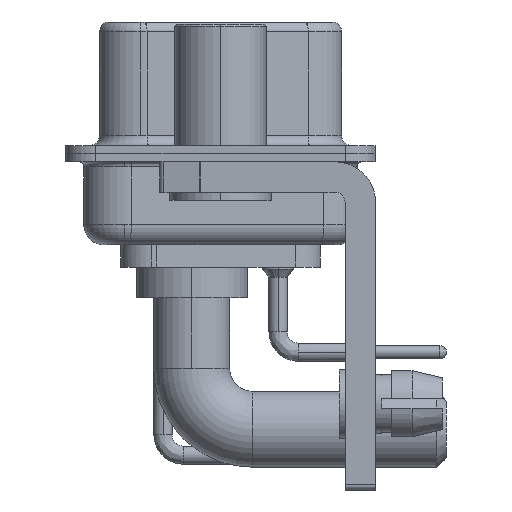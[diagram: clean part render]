
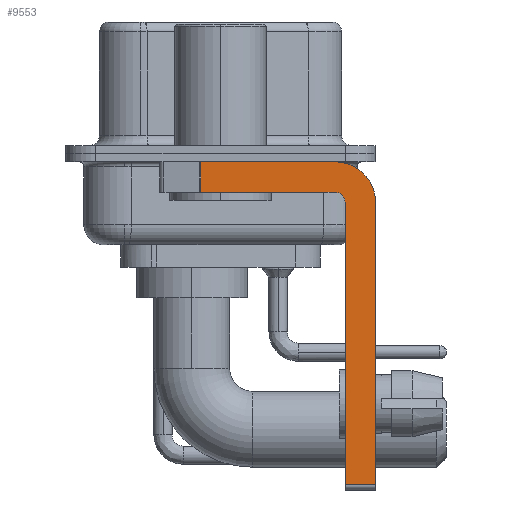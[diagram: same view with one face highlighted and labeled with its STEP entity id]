
A CAD part, left-side view. The second image highlights one B-rep face of the part: STEP entity #9553.
In plain terms, the highlighted planar face has unit normal (-1, 0, 0).
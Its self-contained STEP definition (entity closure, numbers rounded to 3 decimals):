
#256 = DIRECTION ( 'NONE',  ( 0., 0., -1. ) ) ;
#815 = LINE ( 'NONE', #10758, #29738 ) ;
#820 = VERTEX_POINT ( 'NONE', #36194 ) ;
#2617 = CARTESIAN_POINT ( 'NONE',  ( -2.9, 3., -0.4 ) ) ;
#3922 = CARTESIAN_POINT ( 'NONE',  ( -2.9, 0.978, -1.9 ) ) ;
#4291 = CIRCLE ( 'NONE', #25644, 2. ) ;
#4323 = CARTESIAN_POINT ( 'NONE',  ( -2.9, -5.65, -2.4 ) ) ;
#5195 = VERTEX_POINT ( 'NONE', #13333 ) ;
#5649 = CARTESIAN_POINT ( 'NONE',  ( -2.9, -7.65, -2.4 ) ) ;
#6351 = EDGE_CURVE ( 'NONE', #15747, #5195, #4291, .T. ) ;
#7833 = AXIS2_PLACEMENT_3D ( 'NONE', #21275, #9459, #33469 ) ;
#8758 = LINE ( 'NONE', #2617, #20446 ) ;
#9337 = VERTEX_POINT ( 'NONE', #18661 ) ;
#9459 = DIRECTION ( 'NONE',  ( 1., 0., 0. ) ) ;
#9553 = ADVANCED_FACE ( 'NONE', ( #19042 ), #27560, .F. ) ;
#10254 = DIRECTION ( 'NONE',  ( 0., 0., -1. ) ) ;
#10627 = EDGE_CURVE ( 'NONE', #5195, #28362, #17851, .T. ) ;
#10758 = CARTESIAN_POINT ( 'NONE',  ( -2.9, -6.15, -16.6 ) ) ;
#10944 = VECTOR ( 'NONE', #28007, 1000. ) ;
#11276 = EDGE_LOOP ( 'NONE', ( #33305, #21665, #29702, #14302, #29640, #30892, #36954, #36465 ) ) ;
#12974 = CARTESIAN_POINT ( 'NONE',  ( -2.9, -5.65, -2.4 ) ) ;
#13315 = DIRECTION ( 'NONE',  ( 1., 0., 0. ) ) ;
#13333 = CARTESIAN_POINT ( 'NONE',  ( -2.9, -7.65, -2.4 ) ) ;
#13985 = VECTOR ( 'NONE', #28885, 1000. ) ;
#14302 = ORIENTED_EDGE ( 'NONE', *, *, #20305, .F. ) ;
#14846 = DIRECTION ( 'NONE',  ( 0., 0., -1. ) ) ;
#15426 = AXIS2_PLACEMENT_3D ( 'NONE', #12974, #24576, #36221 ) ;
#15747 = VERTEX_POINT ( 'NONE', #36193 ) ;
#16373 = CARTESIAN_POINT ( 'NONE',  ( -2.9, -5.65, -1.9 ) ) ;
#17457 = CARTESIAN_POINT ( 'NONE',  ( -2.9, -5.65, -1.9 ) ) ;
#17851 = LINE ( 'NONE', #5649, #20055 ) ;
#18661 = CARTESIAN_POINT ( 'NONE',  ( -2.9, 0.978, -1.9 ) ) ;
#19042 = FACE_OUTER_BOUND ( 'NONE', #11276, .T. ) ;
#19238 = LINE ( 'NONE', #16373, #10944 ) ;
#19746 = LINE ( 'NONE', #25463, #13985 ) ;
#20055 = VECTOR ( 'NONE', #256, 1000. ) ;
#20305 = EDGE_CURVE ( 'NONE', #28419, #33763, #29396, .T. ) ;
#20446 = VECTOR ( 'NONE', #29334, 1000. ) ;
#20767 = CARTESIAN_POINT ( 'NONE',  ( -2.9, -6.15, -2.4 ) ) ;
#20810 = EDGE_CURVE ( 'NONE', #820, #28362, #19746, .T. ) ;
#21275 = CARTESIAN_POINT ( 'NONE',  ( -2.9, -5.65, -2.4 ) ) ;
#21665 = ORIENTED_EDGE ( 'NONE', *, *, #34606, .T. ) ;
#21956 = VERTEX_POINT ( 'NONE', #24547 ) ;
#24547 = CARTESIAN_POINT ( 'NONE',  ( -2.9, 0.978, -0.4 ) ) ;
#24576 = DIRECTION ( 'NONE',  ( -1., 0., 0. ) ) ;
#25463 = CARTESIAN_POINT ( 'NONE',  ( -2.9, -5.65, -16.35 ) ) ;
#25644 = AXIS2_PLACEMENT_3D ( 'NONE', #4323, #13315, #10254 ) ;
#25975 = EDGE_CURVE ( 'NONE', #820, #28419, #815, .T. ) ;
#27079 = EDGE_CURVE ( 'NONE', #33763, #9337, #19238, .T. ) ;
#27560 = PLANE ( 'NONE',  #7833 ) ;
#27905 = DIRECTION ( 'NONE',  ( 0., 0., 1. ) ) ;
#28007 = DIRECTION ( 'NONE',  ( 0., 1., 0. ) ) ;
#28362 = VERTEX_POINT ( 'NONE', #36991 ) ;
#28419 = VERTEX_POINT ( 'NONE', #20767 ) ;
#28885 = DIRECTION ( 'NONE',  ( 0., -1., 0. ) ) ;
#29334 = DIRECTION ( 'NONE',  ( 0., -1., 0. ) ) ;
#29396 = CIRCLE ( 'NONE', #15426, 0.5 ) ;
#29640 = ORIENTED_EDGE ( 'NONE', *, *, #25975, .F. ) ;
#29702 = ORIENTED_EDGE ( 'NONE', *, *, #27079, .F. ) ;
#29738 = VECTOR ( 'NONE', #27905, 1000. ) ;
#30060 = LINE ( 'NONE', #3922, #34980 ) ;
#30892 = ORIENTED_EDGE ( 'NONE', *, *, #20810, .T. ) ;
#33305 = ORIENTED_EDGE ( 'NONE', *, *, #36340, .F. ) ;
#33469 = DIRECTION ( 'NONE',  ( 0., 0., -1. ) ) ;
#33763 = VERTEX_POINT ( 'NONE', #17457 ) ;
#34606 = EDGE_CURVE ( 'NONE', #21956, #9337, #30060, .T. ) ;
#34980 = VECTOR ( 'NONE', #14846, 1000. ) ;
#36193 = CARTESIAN_POINT ( 'NONE',  ( -2.9, -5.65, -0.4 ) ) ;
#36194 = CARTESIAN_POINT ( 'NONE',  ( -2.9, -6.15, -16.35 ) ) ;
#36221 = DIRECTION ( 'NONE',  ( 0., 0., 1. ) ) ;
#36340 = EDGE_CURVE ( 'NONE', #21956, #15747, #8758, .T. ) ;
#36465 = ORIENTED_EDGE ( 'NONE', *, *, #6351, .F. ) ;
#36954 = ORIENTED_EDGE ( 'NONE', *, *, #10627, .F. ) ;
#36991 = CARTESIAN_POINT ( 'NONE',  ( -2.9, -7.65, -16.35 ) ) ;
